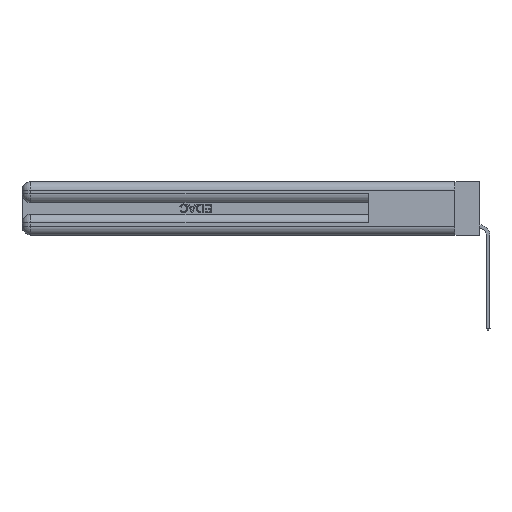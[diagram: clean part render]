
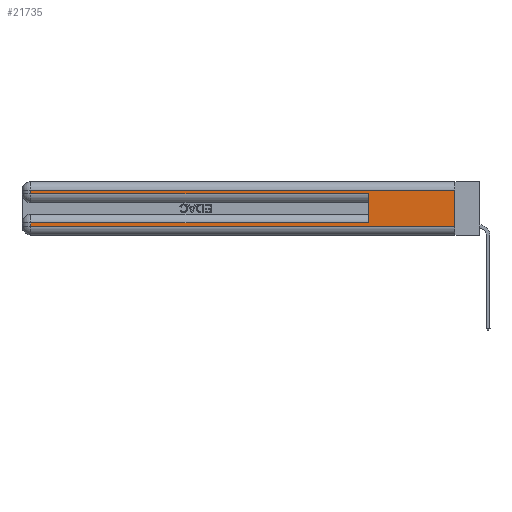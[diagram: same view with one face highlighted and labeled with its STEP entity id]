
A CAD part, left-side view. The second image highlights one B-rep face of the part: STEP entity #21735.
In plain terms, the highlighted planar face has unit normal (-1, 0, 0).
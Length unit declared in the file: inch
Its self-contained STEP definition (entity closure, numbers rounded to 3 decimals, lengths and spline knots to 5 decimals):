
#412 = VERTEX_POINT ( 'NONE', #10388 ) ;
#708 = CARTESIAN_POINT ( 'NONE',  ( 0., 2.94, 0.37 ) ) ;
#807 = ORIENTED_EDGE ( 'NONE', *, *, #3827, .F. ) ;
#1450 = VERTEX_POINT ( 'NONE', #15346 ) ;
#1891 = DIRECTION ( 'NONE',  ( 0., -1., 0. ) ) ;
#2920 = ORIENTED_EDGE ( 'NONE', *, *, #26139, .T. ) ;
#3751 = LINE ( 'NONE', #24049, #28368 ) ;
#3827 = EDGE_CURVE ( 'NONE', #1450, #10714, #28403, .T. ) ;
#4012 = EDGE_CURVE ( 'NONE', #20789, #4780, #25797, .T. ) ;
#4712 = EDGE_CURVE ( 'NONE', #29037, #10714, #12002, .T. ) ;
#4780 = VERTEX_POINT ( 'NONE', #23765 ) ;
#5177 = VECTOR ( 'NONE', #15247, 39.37008 ) ;
#5513 = VECTOR ( 'NONE', #8852, 39.37008 ) ;
#5948 = LINE ( 'NONE', #708, #5177 ) ;
#6141 = CARTESIAN_POINT ( 'NONE',  ( 0., 0., 0.37 ) ) ;
#6681 = CARTESIAN_POINT ( 'NONE',  ( 0., 0., 0.285 ) ) ;
#6707 = EDGE_CURVE ( 'NONE', #1450, #26363, #8134, .T. ) ;
#7105 = ORIENTED_EDGE ( 'NONE', *, *, #28082, .T. ) ;
#7218 = CARTESIAN_POINT ( 'NONE',  ( 0., 0., 0.37 ) ) ;
#7796 = CARTESIAN_POINT ( 'NONE',  ( 0., 2.94, 0.285 ) ) ;
#8134 = LINE ( 'NONE', #19071, #20083 ) ;
#8228 = EDGE_CURVE ( 'NONE', #20789, #412, #3751, .T. ) ;
#8852 = DIRECTION ( 'NONE',  ( 0., 0., -1. ) ) ;
#9586 = EDGE_LOOP ( 'NONE', ( #807, #20975, #7105, #2920, #16731, #19212, #26976, #28406 ) ) ;
#9629 = DIRECTION ( 'NONE',  ( 0., 0., -1. ) ) ;
#10388 = CARTESIAN_POINT ( 'NONE',  ( 0., 0.6, 0.285 ) ) ;
#10714 = VERTEX_POINT ( 'NONE', #18429 ) ;
#11109 = CARTESIAN_POINT ( 'NONE',  ( 0., 0., 0.085 ) ) ;
#11259 = VECTOR ( 'NONE', #26017, 39.37008 ) ;
#12002 = LINE ( 'NONE', #16479, #11259 ) ;
#12198 = DIRECTION ( 'NONE',  ( 0., 0., 1. ) ) ;
#13390 = AXIS2_PLACEMENT_3D ( 'NONE', #7218, #23900, #9629 ) ;
#13521 = FACE_OUTER_BOUND ( 'NONE', #9586, .T. ) ;
#14308 = PLANE ( 'NONE',  #13390 ) ;
#15247 = DIRECTION ( 'NONE',  ( 0., 0., -1. ) ) ;
#15338 = VERTEX_POINT ( 'NONE', #7796 ) ;
#15346 = CARTESIAN_POINT ( 'NONE',  ( 0., 0., 0.31 ) ) ;
#15628 = DIRECTION ( 'NONE',  ( 0., 0., -1. ) ) ;
#15879 = DIRECTION ( 'NONE',  ( 0., 1., 0. ) ) ;
#16047 = CARTESIAN_POINT ( 'NONE',  ( 0., 2.94, 0.37 ) ) ;
#16479 = CARTESIAN_POINT ( 'NONE',  ( 0., 0., 0.06 ) ) ;
#16731 = ORIENTED_EDGE ( 'NONE', *, *, #8228, .F. ) ;
#17382 = VECTOR ( 'NONE', #1891, 39.37008 ) ;
#17442 = CARTESIAN_POINT ( 'NONE',  ( 0., 2.94, 0.06 ) ) ;
#18071 = EDGE_CURVE ( 'NONE', #4780, #29037, #5948, .T. ) ;
#18382 = VECTOR ( 'NONE', #15628, 39.37008 ) ;
#18429 = CARTESIAN_POINT ( 'NONE',  ( 0., 0., 0.06 ) ) ;
#19071 = CARTESIAN_POINT ( 'NONE',  ( 0., 0., 0.31 ) ) ;
#19212 = ORIENTED_EDGE ( 'NONE', *, *, #4012, .T. ) ;
#19494 = VECTOR ( 'NONE', #15879, 39.37008 ) ;
#20083 = VECTOR ( 'NONE', #21468, 39.37008 ) ;
#20789 = VERTEX_POINT ( 'NONE', #30633 ) ;
#20975 = ORIENTED_EDGE ( 'NONE', *, *, #6707, .T. ) ;
#21468 = DIRECTION ( 'NONE',  ( 0., 1., 0. ) ) ;
#21735 = ADVANCED_FACE ( 'NONE', ( #13521 ), #14308, .F. ) ;
#23765 = CARTESIAN_POINT ( 'NONE',  ( 0., 2.94, 0.085 ) ) ;
#23900 = DIRECTION ( 'NONE',  ( 1., 0., 0. ) ) ;
#24049 = CARTESIAN_POINT ( 'NONE',  ( 0., 0.6, 0.145 ) ) ;
#24279 = CARTESIAN_POINT ( 'NONE',  ( 0., 2.94, 0.31 ) ) ;
#24442 = LINE ( 'NONE', #6681, #17382 ) ;
#25797 = LINE ( 'NONE', #11109, #19494 ) ;
#26017 = DIRECTION ( 'NONE',  ( 0., -1., 0. ) ) ;
#26139 = EDGE_CURVE ( 'NONE', #15338, #412, #24442, .T. ) ;
#26363 = VERTEX_POINT ( 'NONE', #24279 ) ;
#26976 = ORIENTED_EDGE ( 'NONE', *, *, #18071, .T. ) ;
#28082 = EDGE_CURVE ( 'NONE', #26363, #15338, #29338, .T. ) ;
#28368 = VECTOR ( 'NONE', #12198, 39.37008 ) ;
#28403 = LINE ( 'NONE', #6141, #18382 ) ;
#28406 = ORIENTED_EDGE ( 'NONE', *, *, #4712, .T. ) ;
#29037 = VERTEX_POINT ( 'NONE', #17442 ) ;
#29338 = LINE ( 'NONE', #16047, #5513 ) ;
#30633 = CARTESIAN_POINT ( 'NONE',  ( 0., 0.6, 0.085 ) ) ;
